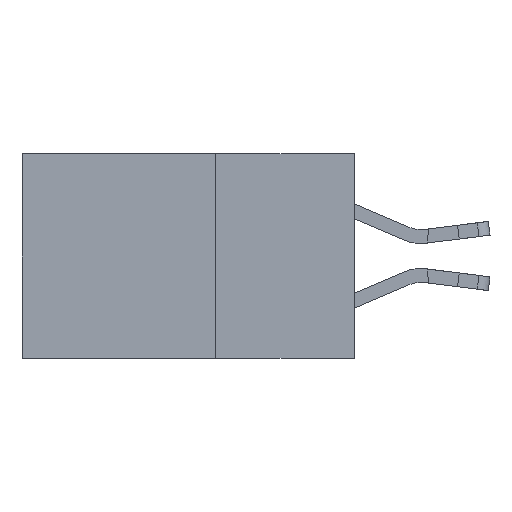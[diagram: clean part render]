
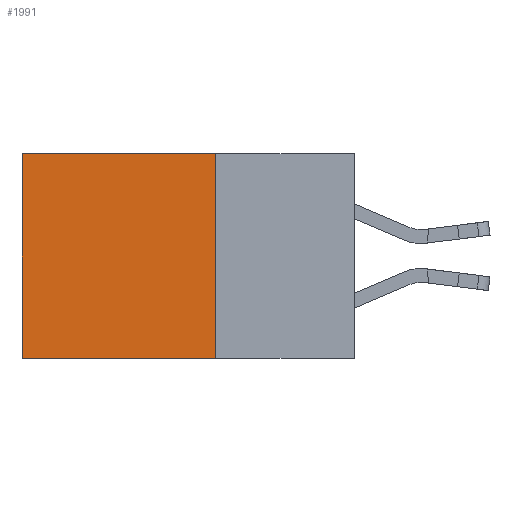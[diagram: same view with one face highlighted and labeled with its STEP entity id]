
A CAD part, left-side view. The second image highlights one B-rep face of the part: STEP entity #1991.
In plain terms, the highlighted planar face has unit normal (-1, 0, 0).
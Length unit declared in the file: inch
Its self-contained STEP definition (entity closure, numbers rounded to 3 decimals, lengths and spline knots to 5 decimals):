
#1102 = DIRECTION ( 'NONE',  ( 0., 1., 0. ) ) ;
#1991 = ADVANCED_FACE ( 'NONE', ( #10174 ), #16604, .F. ) ;
#2121 = CARTESIAN_POINT ( 'NONE',  ( 0.2615, 0.25, -0.37 ) ) ;
#2327 = CARTESIAN_POINT ( 'NONE',  ( 0.2615, 0.6, -0.37 ) ) ;
#3113 = DIRECTION ( 'NONE',  ( 0., 0., -1. ) ) ;
#3461 = AXIS2_PLACEMENT_3D ( 'NONE', #2121, #15008, #3113 ) ;
#4009 = LINE ( 'NONE', #2327, #11451 ) ;
#5174 = VERTEX_POINT ( 'NONE', #18481 ) ;
#5466 = CARTESIAN_POINT ( 'NONE',  ( 0.2615, 0.25, -0.37 ) ) ;
#6147 = VERTEX_POINT ( 'NONE', #13581 ) ;
#8967 = VECTOR ( 'NONE', #1102, 39.37008 ) ;
#8984 = VERTEX_POINT ( 'NONE', #12763 ) ;
#10087 = EDGE_CURVE ( 'NONE', #5174, #8984, #4009, .T. ) ;
#10174 = FACE_OUTER_BOUND ( 'NONE', #17371, .T. ) ;
#10528 = DIRECTION ( 'NONE',  ( 0., 0., -1. ) ) ;
#10553 = LINE ( 'NONE', #20352, #12741 ) ;
#10569 = ORIENTED_EDGE ( 'NONE', *, *, #14653, .T. ) ;
#11451 = VECTOR ( 'NONE', #13321, 39.37008 ) ;
#11823 = VERTEX_POINT ( 'NONE', #17742 ) ;
#12161 = EDGE_CURVE ( 'NONE', #11823, #8984, #10553, .T. ) ;
#12288 = ORIENTED_EDGE ( 'NONE', *, *, #10087, .T. ) ;
#12741 = VECTOR ( 'NONE', #17304, 39.37008 ) ;
#12763 = CARTESIAN_POINT ( 'NONE',  ( 0.2615, 0.6, -0.37 ) ) ;
#13321 = DIRECTION ( 'NONE',  ( 0., 0., -1. ) ) ;
#13581 = CARTESIAN_POINT ( 'NONE',  ( 0.2615, 0.25, 0. ) ) ;
#14653 = EDGE_CURVE ( 'NONE', #6147, #5174, #19061, .T. ) ;
#15008 = DIRECTION ( 'NONE',  ( 1., 0., 0. ) ) ;
#15167 = LINE ( 'NONE', #5466, #17690 ) ;
#16604 = PLANE ( 'NONE',  #3461 ) ;
#17304 = DIRECTION ( 'NONE',  ( 0., 1., 0. ) ) ;
#17371 = EDGE_LOOP ( 'NONE', ( #12288, #19631, #19830, #10569 ) ) ;
#17504 = EDGE_CURVE ( 'NONE', #6147, #11823, #15167, .T. ) ;
#17690 = VECTOR ( 'NONE', #10528, 39.37008 ) ;
#17742 = CARTESIAN_POINT ( 'NONE',  ( 0.2615, 0.25, -0.37 ) ) ;
#18481 = CARTESIAN_POINT ( 'NONE',  ( 0.2615, 0.6, 0. ) ) ;
#18953 = CARTESIAN_POINT ( 'NONE',  ( 0.2615, 0.25, 0. ) ) ;
#19061 = LINE ( 'NONE', #18953, #8967 ) ;
#19631 = ORIENTED_EDGE ( 'NONE', *, *, #12161, .F. ) ;
#19830 = ORIENTED_EDGE ( 'NONE', *, *, #17504, .F. ) ;
#20352 = CARTESIAN_POINT ( 'NONE',  ( 0.2615, 0.25, -0.37 ) ) ;
